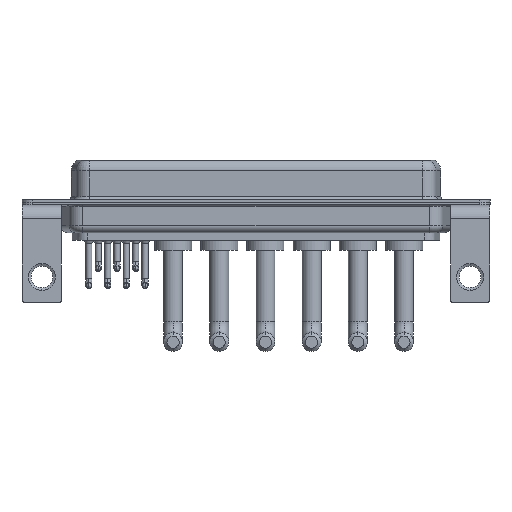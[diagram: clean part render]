
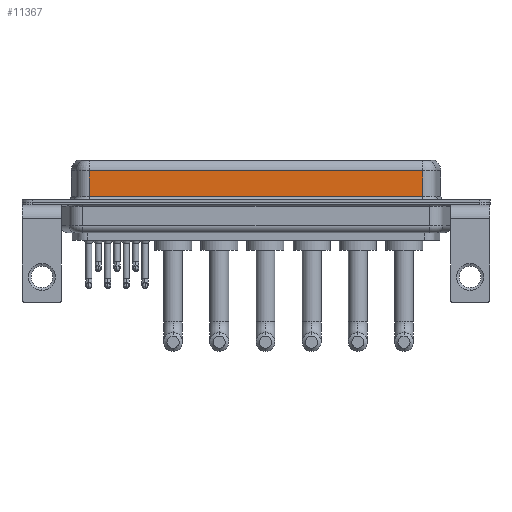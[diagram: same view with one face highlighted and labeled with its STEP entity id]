
A CAD part, front view. The second image highlights one B-rep face of the part: STEP entity #11367.
In plain terms, the highlighted planar face has unit normal (0, -1, 0).
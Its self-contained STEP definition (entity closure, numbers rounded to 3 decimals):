
#138 = VERTEX_POINT ( 'NONE', #8390 ) ;
#1027 = CARTESIAN_POINT ( 'NONE',  ( 56.462, -3.95, 4.65 ) ) ;
#1391 = DIRECTION ( 'NONE',  ( 0., 0., 1. ) ) ;
#2221 = EDGE_CURVE ( 'NONE', #10512, #138, #11765, .T. ) ;
#3162 = CARTESIAN_POINT ( 'NONE',  ( 56.462, -3.95, 4.65 ) ) ;
#3264 = LINE ( 'NONE', #13543, #15476 ) ;
#4657 = VERTEX_POINT ( 'NONE', #1027 ) ;
#5775 = PLANE ( 'NONE',  #17136 ) ;
#6082 = DIRECTION ( 'NONE',  ( -1., 0., 0. ) ) ;
#6440 = EDGE_CURVE ( 'NONE', #138, #12952, #3264, .T. ) ;
#6548 = ORIENTED_EDGE ( 'NONE', *, *, #17210, .T. ) ;
#6793 = ORIENTED_EDGE ( 'NONE', *, *, #18223, .F. ) ;
#6942 = VECTOR ( 'NONE', #10292, 1000. ) ;
#8390 = CARTESIAN_POINT ( 'NONE',  ( 7.038, -3.95, 0.9 ) ) ;
#9355 = LINE ( 'NONE', #3162, #16328 ) ;
#10292 = DIRECTION ( 'NONE',  ( 0., 0., -1. ) ) ;
#10512 = VERTEX_POINT ( 'NONE', #14776 ) ;
#11367 = ADVANCED_FACE ( 'NONE', ( #14780 ), #5775, .F. ) ;
#11689 = DIRECTION ( 'NONE',  ( 0., 1., 0. ) ) ;
#11765 = LINE ( 'NONE', #17676, #6942 ) ;
#12209 = EDGE_LOOP ( 'NONE', ( #6793, #6548, #14145, #14149 ) ) ;
#12952 = VERTEX_POINT ( 'NONE', #18007 ) ;
#13543 = CARTESIAN_POINT ( 'NONE',  ( 56.462, -3.95, 0.9 ) ) ;
#14145 = ORIENTED_EDGE ( 'NONE', *, *, #2221, .T. ) ;
#14149 = ORIENTED_EDGE ( 'NONE', *, *, #6440, .T. ) ;
#14501 = VECTOR ( 'NONE', #18333, 1000. ) ;
#14776 = CARTESIAN_POINT ( 'NONE',  ( 7.038, -3.95, 4.65 ) ) ;
#14780 = FACE_OUTER_BOUND ( 'NONE', #12209, .T. ) ;
#15181 = DIRECTION ( 'NONE',  ( 1., 0., 0. ) ) ;
#15238 = CARTESIAN_POINT ( 'NONE',  ( 56.462, -3.95, 6.4 ) ) ;
#15476 = VECTOR ( 'NONE', #15181, 1000. ) ;
#16328 = VECTOR ( 'NONE', #6082, 1000. ) ;
#17136 = AXIS2_PLACEMENT_3D ( 'NONE', #19153, #11689, #1391 ) ;
#17210 = EDGE_CURVE ( 'NONE', #4657, #10512, #9355, .T. ) ;
#17676 = CARTESIAN_POINT ( 'NONE',  ( 7.038, -3.95, 6.4 ) ) ;
#18007 = CARTESIAN_POINT ( 'NONE',  ( 56.462, -3.95, 0.9 ) ) ;
#18223 = EDGE_CURVE ( 'NONE', #4657, #12952, #18241, .T. ) ;
#18241 = LINE ( 'NONE', #15238, #14501 ) ;
#18333 = DIRECTION ( 'NONE',  ( 0., 0., -1. ) ) ;
#19153 = CARTESIAN_POINT ( 'NONE',  ( 56.462, -3.95, 6.4 ) ) ;
